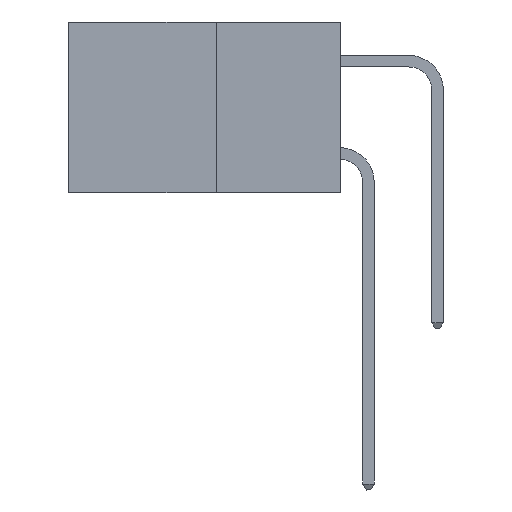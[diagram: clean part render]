
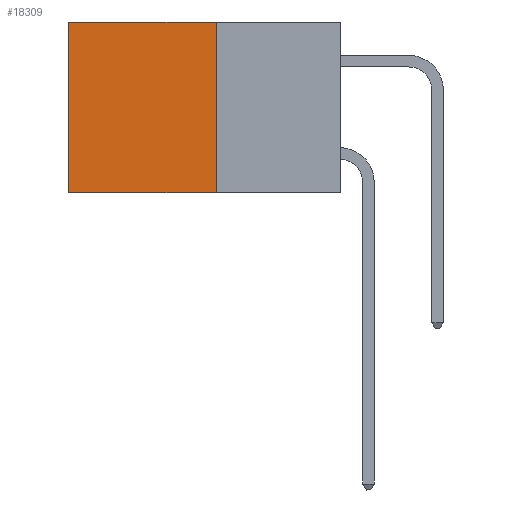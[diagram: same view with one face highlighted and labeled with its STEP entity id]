
A CAD part, left-side view. The second image highlights one B-rep face of the part: STEP entity #18309.
In plain terms, the highlighted planar face has unit normal (-1, 0, 0).
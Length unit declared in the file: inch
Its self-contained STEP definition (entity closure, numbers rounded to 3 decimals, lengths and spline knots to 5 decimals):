
#2035 = DIRECTION ( 'NONE',  ( 0., 0., -1. ) ) ;
#2659 = VERTEX_POINT ( 'NONE', #28357 ) ;
#3107 = LINE ( 'NONE', #15426, #9379 ) ;
#5738 = CARTESIAN_POINT ( 'NONE',  ( 0.277, 0.27, 0. ) ) ;
#5970 = AXIS2_PLACEMENT_3D ( 'NONE', #7658, #10374, #28935 ) ;
#6586 = VERTEX_POINT ( 'NONE', #16898 ) ;
#6778 = VECTOR ( 'NONE', #13848, 39.37008 ) ;
#7658 = CARTESIAN_POINT ( 'NONE',  ( 0.277, 0.27, -0.37 ) ) ;
#8635 = CARTESIAN_POINT ( 'NONE',  ( 0.277, 0.27, -0.37 ) ) ;
#9379 = VECTOR ( 'NONE', #2035, 39.37008 ) ;
#10374 = DIRECTION ( 'NONE',  ( 1., 0., 0. ) ) ;
#10859 = ORIENTED_EDGE ( 'NONE', *, *, #23564, .F. ) ;
#12652 = VERTEX_POINT ( 'NONE', #30270 ) ;
#12985 = ORIENTED_EDGE ( 'NONE', *, *, #17231, .T. ) ;
#13724 = ORIENTED_EDGE ( 'NONE', *, *, #14631, .T. ) ;
#13848 = DIRECTION ( 'NONE',  ( 0., 1., 0. ) ) ;
#14427 = ORIENTED_EDGE ( 'NONE', *, *, #28768, .F. ) ;
#14631 = EDGE_CURVE ( 'NONE', #2659, #24368, #31096, .T. ) ;
#14773 = LINE ( 'NONE', #5738, #6778 ) ;
#14783 = LINE ( 'NONE', #8635, #34119 ) ;
#15426 = CARTESIAN_POINT ( 'NONE',  ( 0.277, 0.27, -0.37 ) ) ;
#16637 = DIRECTION ( 'NONE',  ( 0., 0., -1. ) ) ;
#16898 = CARTESIAN_POINT ( 'NONE',  ( 0.277, 0.27, -0.37 ) ) ;
#17044 = VECTOR ( 'NONE', #16637, 39.37008 ) ;
#17231 = EDGE_CURVE ( 'NONE', #12652, #2659, #14773, .T. ) ;
#18309 = ADVANCED_FACE ( 'NONE', ( #29177 ), #23632, .F. ) ;
#22465 = CARTESIAN_POINT ( 'NONE',  ( 0.277, 0.59, -0.37 ) ) ;
#23282 = EDGE_LOOP ( 'NONE', ( #13724, #10859, #14427, #12985 ) ) ;
#23564 = EDGE_CURVE ( 'NONE', #6586, #24368, #14783, .T. ) ;
#23632 = PLANE ( 'NONE',  #5970 ) ;
#24368 = VERTEX_POINT ( 'NONE', #22465 ) ;
#27237 = DIRECTION ( 'NONE',  ( 0., 1., 0. ) ) ;
#27287 = CARTESIAN_POINT ( 'NONE',  ( 0.277, 0.59, -0.37 ) ) ;
#28357 = CARTESIAN_POINT ( 'NONE',  ( 0.277, 0.59, 0. ) ) ;
#28768 = EDGE_CURVE ( 'NONE', #12652, #6586, #3107, .T. ) ;
#28935 = DIRECTION ( 'NONE',  ( 0., 0., -1. ) ) ;
#29177 = FACE_OUTER_BOUND ( 'NONE', #23282, .T. ) ;
#30270 = CARTESIAN_POINT ( 'NONE',  ( 0.277, 0.27, 0. ) ) ;
#31096 = LINE ( 'NONE', #27287, #17044 ) ;
#34119 = VECTOR ( 'NONE', #27237, 39.37008 ) ;
